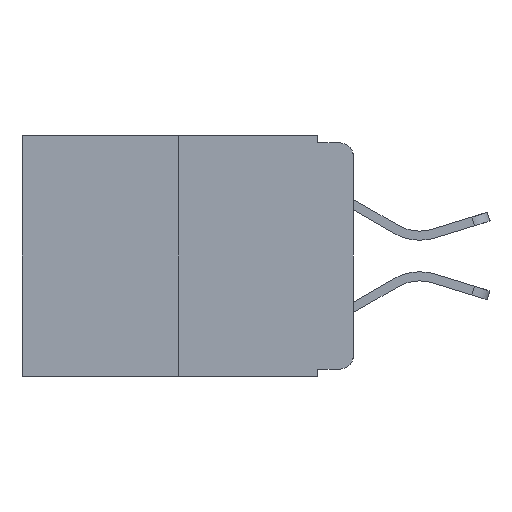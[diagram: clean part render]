
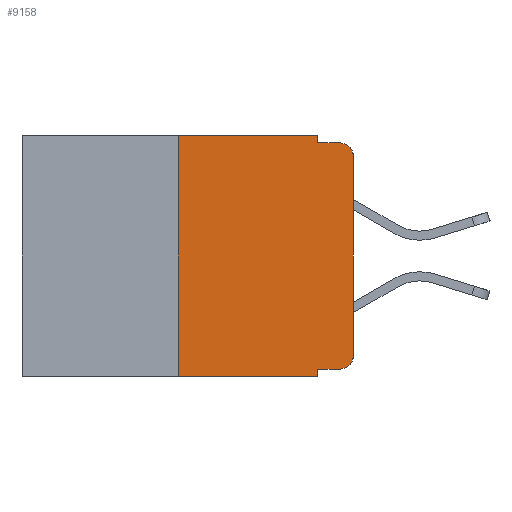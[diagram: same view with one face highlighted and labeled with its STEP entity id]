
A CAD part, left-side view. The second image highlights one B-rep face of the part: STEP entity #9158.
In plain terms, the highlighted planar face has unit normal (-1, 0, 0).
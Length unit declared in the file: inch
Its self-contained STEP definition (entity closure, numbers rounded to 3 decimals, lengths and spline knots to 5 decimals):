
#100 = AXIS2_PLACEMENT_3D ( 'NONE', #12146, #6446, #13055 ) ;
#434 = LINE ( 'NONE', #8899, #11493 ) ;
#822 = EDGE_CURVE ( 'NONE', #11491, #10088, #7184, .T. ) ;
#827 = VECTOR ( 'NONE', #5788, 39.37008 ) ;
#983 = EDGE_CURVE ( 'NONE', #11491, #5110, #7011, .T. ) ;
#986 = EDGE_CURVE ( 'NONE', #1845, #2739, #1226, .T. ) ;
#1003 = EDGE_CURVE ( 'NONE', #6713, #3177, #434, .T. ) ;
#1024 = EDGE_CURVE ( 'NONE', #3316, #6713, #5473, .T. ) ;
#1044 = EDGE_CURVE ( 'NONE', #12144, #3177, #1817, .T. ) ;
#1049 = EDGE_CURVE ( 'NONE', #2407, #12144, #9818, .T. ) ;
#1168 = EDGE_CURVE ( 'NONE', #1845, #5110, #11768, .T. ) ;
#1188 = ORIENTED_EDGE ( 'NONE', *, *, #1049, .T. ) ;
#1226 = LINE ( 'NONE', #5902, #6693 ) ;
#1649 = ORIENTED_EDGE ( 'NONE', *, *, #3748, .F. ) ;
#1664 = ORIENTED_EDGE ( 'NONE', *, *, #1044, .T. ) ;
#1817 = CIRCLE ( 'NONE', #12323, 0.02 ) ;
#1845 = VERTEX_POINT ( 'NONE', #9162 ) ;
#2125 = CARTESIAN_POINT ( 'NONE',  ( 0., 0.473, -0.343 ) ) ;
#2407 = VERTEX_POINT ( 'NONE', #13165 ) ;
#2673 = DIRECTION ( 'NONE',  ( 0., -1., 0. ) ) ;
#2709 = CARTESIAN_POINT ( 'NONE',  ( 0., 0.051, 0. ) ) ;
#2739 = VERTEX_POINT ( 'NONE', #11279 ) ;
#2882 = CARTESIAN_POINT ( 'NONE',  ( 0., 0.02, -0.313 ) ) ;
#3016 = DIRECTION ( 'NONE',  ( 0., 0., 1. ) ) ;
#3038 = DIRECTION ( 'NONE',  ( 0., 0., -1. ) ) ;
#3177 = VERTEX_POINT ( 'NONE', #12711 ) ;
#3316 = VERTEX_POINT ( 'NONE', #11361 ) ;
#3472 = ORIENTED_EDGE ( 'NONE', *, *, #1168, .T. ) ;
#3711 = CARTESIAN_POINT ( 'NONE',  ( 0., 0.051, -0.343 ) ) ;
#3748 = EDGE_CURVE ( 'NONE', #2739, #3316, #8538, .T. ) ;
#4066 = DIRECTION ( 'NONE',  ( 0., 0., -1. ) ) ;
#4114 = DIRECTION ( 'NONE',  ( 0., -1., 0. ) ) ;
#4382 = ORIENTED_EDGE ( 'NONE', *, *, #983, .F. ) ;
#4796 = ORIENTED_EDGE ( 'NONE', *, *, #986, .F. ) ;
#4832 = CARTESIAN_POINT ( 'NONE',  ( 0., 0.02, -0.333 ) ) ;
#5074 = CARTESIAN_POINT ( 'NONE',  ( 0., 0.02, -0.03 ) ) ;
#5110 = VERTEX_POINT ( 'NONE', #3711 ) ;
#5373 = ORIENTED_EDGE ( 'NONE', *, *, #822, .T. ) ;
#5473 = LINE ( 'NONE', #11233, #8120 ) ;
#5659 = CIRCLE ( 'NONE', #12853, 0.02 ) ;
#5788 = DIRECTION ( 'NONE',  ( 0., -1., 0. ) ) ;
#5868 = VECTOR ( 'NONE', #2673, 39.37008 ) ;
#5902 = CARTESIAN_POINT ( 'NONE',  ( 0., 0.25, 0. ) ) ;
#6446 = DIRECTION ( 'NONE',  ( 1., 0., 0. ) ) ;
#6470 = DIRECTION ( 'NONE',  ( 0., 0., -1. ) ) ;
#6599 = CARTESIAN_POINT ( 'NONE',  ( 0., 0., -0.03 ) ) ;
#6643 = CARTESIAN_POINT ( 'NONE',  ( 0., 0., 0. ) ) ;
#6693 = VECTOR ( 'NONE', #8328, 39.37008 ) ;
#6713 = VERTEX_POINT ( 'NONE', #11425 ) ;
#7011 = LINE ( 'NONE', #2709, #11784 ) ;
#7184 = LINE ( 'NONE', #11208, #9519 ) ;
#7302 = ORIENTED_EDGE ( 'NONE', *, *, #1024, .F. ) ;
#7375 = ORIENTED_EDGE ( 'NONE', *, *, #1003, .F. ) ;
#7473 = ORIENTED_EDGE ( 'NONE', *, *, #7975, .T. ) ;
#7975 = EDGE_CURVE ( 'NONE', #10088, #2407, #5659, .T. ) ;
#8120 = VECTOR ( 'NONE', #10234, 39.37008 ) ;
#8328 = DIRECTION ( 'NONE',  ( 0., 0., 1. ) ) ;
#8538 = LINE ( 'NONE', #11586, #5868 ) ;
#8899 = CARTESIAN_POINT ( 'NONE',  ( 0., 0.051, -0.01 ) ) ;
#9158 = ADVANCED_FACE ( 'NONE', ( #12904 ), #10359, .F. ) ;
#9162 = CARTESIAN_POINT ( 'NONE',  ( 0., 0.25, -0.343 ) ) ;
#9501 = VECTOR ( 'NONE', #3016, 39.37008 ) ;
#9519 = VECTOR ( 'NONE', #4114, 39.37008 ) ;
#9818 = LINE ( 'NONE', #6643, #9501 ) ;
#9840 = DIRECTION ( 'NONE',  ( -1., 0., 0. ) ) ;
#9979 = DIRECTION ( 'NONE',  ( -1., 0., 0. ) ) ;
#10088 = VERTEX_POINT ( 'NONE', #4832 ) ;
#10234 = DIRECTION ( 'NONE',  ( 0., 0., -1. ) ) ;
#10359 = PLANE ( 'NONE',  #100 ) ;
#10908 = CARTESIAN_POINT ( 'NONE',  ( 0., 0.051, -0.333 ) ) ;
#11203 = EDGE_LOOP ( 'NONE', ( #1188, #1664, #7375, #7302, #1649, #4796, #3472, #4382, #5373, #7473 ) ) ;
#11208 = CARTESIAN_POINT ( 'NONE',  ( 0., 0.051, -0.333 ) ) ;
#11233 = CARTESIAN_POINT ( 'NONE',  ( 0., 0.051, 0. ) ) ;
#11279 = CARTESIAN_POINT ( 'NONE',  ( 0., 0.25, 0. ) ) ;
#11361 = CARTESIAN_POINT ( 'NONE',  ( 0., 0.051, 0. ) ) ;
#11425 = CARTESIAN_POINT ( 'NONE',  ( 0., 0.051, -0.01 ) ) ;
#11491 = VERTEX_POINT ( 'NONE', #10908 ) ;
#11493 = VECTOR ( 'NONE', #13272, 39.37008 ) ;
#11586 = CARTESIAN_POINT ( 'NONE',  ( 0., 0.473, 0. ) ) ;
#11768 = LINE ( 'NONE', #2125, #827 ) ;
#11784 = VECTOR ( 'NONE', #6470, 39.37008 ) ;
#12144 = VERTEX_POINT ( 'NONE', #6599 ) ;
#12146 = CARTESIAN_POINT ( 'NONE',  ( 0., 0.473, 0. ) ) ;
#12323 = AXIS2_PLACEMENT_3D ( 'NONE', #5074, #9840, #3038 ) ;
#12711 = CARTESIAN_POINT ( 'NONE',  ( 0., 0.02, -0.01 ) ) ;
#12853 = AXIS2_PLACEMENT_3D ( 'NONE', #2882, #9979, #4066 ) ;
#12904 = FACE_OUTER_BOUND ( 'NONE', #11203, .T. ) ;
#13055 = DIRECTION ( 'NONE',  ( 0., 0., -1. ) ) ;
#13165 = CARTESIAN_POINT ( 'NONE',  ( 0., 0., -0.313 ) ) ;
#13272 = DIRECTION ( 'NONE',  ( 0., -1., 0. ) ) ;
